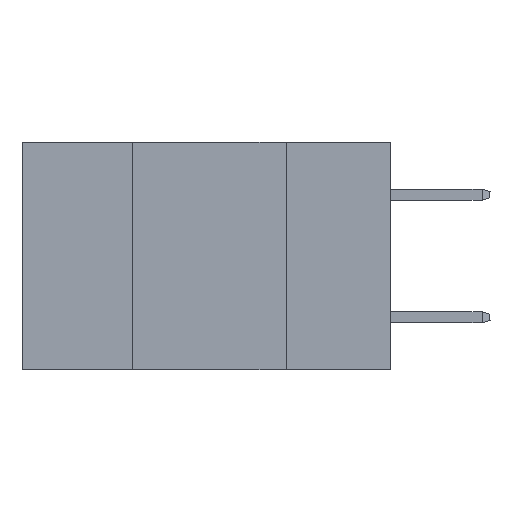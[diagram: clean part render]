
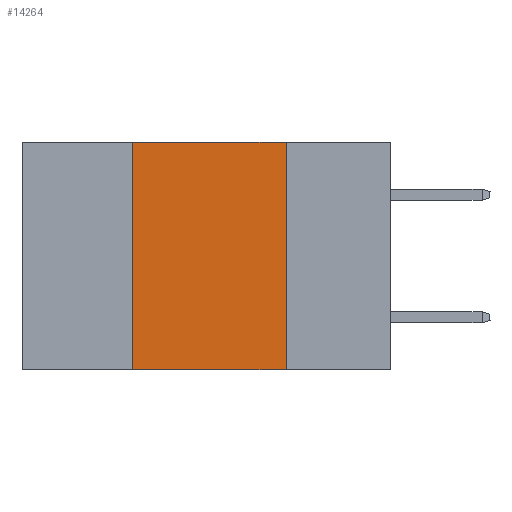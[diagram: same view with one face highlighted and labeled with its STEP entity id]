
A CAD part, left-side view. The second image highlights one B-rep face of the part: STEP entity #14264.
In plain terms, the highlighted planar face has unit normal (-1, 0, 0).
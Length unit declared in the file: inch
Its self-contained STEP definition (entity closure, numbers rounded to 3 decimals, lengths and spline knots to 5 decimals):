
#592 = DIRECTION ( 'NONE',  ( 1., 0., 0. ) ) ;
#1150 = CARTESIAN_POINT ( 'NONE',  ( 0., 0.17, 0. ) ) ;
#1489 = EDGE_CURVE ( 'NONE', #30698, #14853, #22600, .T. ) ;
#2473 = CARTESIAN_POINT ( 'NONE',  ( 0., 0.6, -0.37 ) ) ;
#4148 = VECTOR ( 'NONE', #12597, 39.37008 ) ;
#4633 = EDGE_CURVE ( 'NONE', #22029, #14853, #17815, .T. ) ;
#6428 = FACE_OUTER_BOUND ( 'NONE', #35384, .T. ) ;
#6756 = CARTESIAN_POINT ( 'NONE',  ( 0., 0.42, 0. ) ) ;
#8754 = VECTOR ( 'NONE', #15723, 39.37008 ) ;
#8800 = VECTOR ( 'NONE', #20845, 39.37008 ) ;
#10517 = VERTEX_POINT ( 'NONE', #11237 ) ;
#10645 = ORIENTED_EDGE ( 'NONE', *, *, #1489, .T. ) ;
#11237 = CARTESIAN_POINT ( 'NONE',  ( 0., 0.42, 0. ) ) ;
#11915 = LINE ( 'NONE', #33004, #8754 ) ;
#12597 = DIRECTION ( 'NONE',  ( 0., 0., -1. ) ) ;
#13313 = LINE ( 'NONE', #6756, #8800 ) ;
#14264 = ADVANCED_FACE ( 'NONE', ( #6428 ), #28604, .F. ) ;
#14853 = VERTEX_POINT ( 'NONE', #27095 ) ;
#15549 = CARTESIAN_POINT ( 'NONE',  ( 0., 0.17, 0. ) ) ;
#15723 = DIRECTION ( 'NONE',  ( 0., -1., 0. ) ) ;
#17569 = CARTESIAN_POINT ( 'NONE',  ( 0., 0.6, 0. ) ) ;
#17815 = LINE ( 'NONE', #1150, #4148 ) ;
#18494 = ORIENTED_EDGE ( 'NONE', *, *, #4633, .F. ) ;
#19622 = CARTESIAN_POINT ( 'NONE',  ( 0., 0.42, -0.37 ) ) ;
#20845 = DIRECTION ( 'NONE',  ( 0., 0., 1. ) ) ;
#22029 = VERTEX_POINT ( 'NONE', #15549 ) ;
#22600 = LINE ( 'NONE', #2473, #31685 ) ;
#24105 = DIRECTION ( 'NONE',  ( 0., 0., -1. ) ) ;
#24884 = EDGE_CURVE ( 'NONE', #30698, #10517, #13313, .T. ) ;
#27052 = ORIENTED_EDGE ( 'NONE', *, *, #31629, .F. ) ;
#27095 = CARTESIAN_POINT ( 'NONE',  ( 0., 0.17, -0.37 ) ) ;
#28118 = DIRECTION ( 'NONE',  ( 0., -1., 0. ) ) ;
#28604 = PLANE ( 'NONE',  #33250 ) ;
#28681 = ORIENTED_EDGE ( 'NONE', *, *, #24884, .F. ) ;
#30698 = VERTEX_POINT ( 'NONE', #19622 ) ;
#31629 = EDGE_CURVE ( 'NONE', #10517, #22029, #11915, .T. ) ;
#31685 = VECTOR ( 'NONE', #28118, 39.37008 ) ;
#33004 = CARTESIAN_POINT ( 'NONE',  ( 0., 0.6, 0. ) ) ;
#33250 = AXIS2_PLACEMENT_3D ( 'NONE', #17569, #592, #24105 ) ;
#35384 = EDGE_LOOP ( 'NONE', ( #18494, #27052, #28681, #10645 ) ) ;
